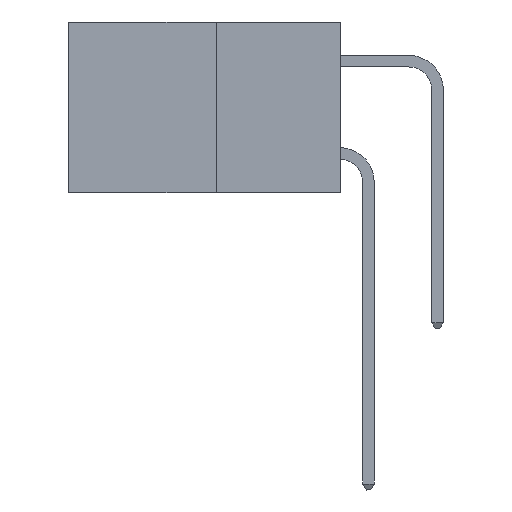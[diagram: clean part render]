
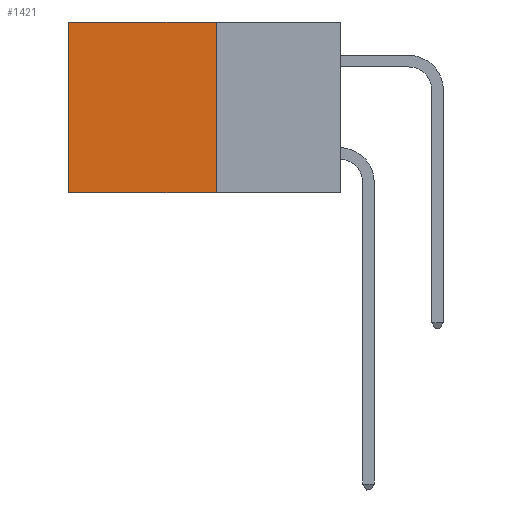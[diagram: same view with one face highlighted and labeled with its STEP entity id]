
A CAD part, left-side view. The second image highlights one B-rep face of the part: STEP entity #1421.
In plain terms, the highlighted planar face has unit normal (-1, 0, 0).
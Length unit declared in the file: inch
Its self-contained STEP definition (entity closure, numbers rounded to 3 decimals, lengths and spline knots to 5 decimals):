
#154 = DIRECTION ( 'NONE',  ( 0., 0., -1. ) ) ;
#242 = ORIENTED_EDGE ( 'NONE', *, *, #6217, .T. ) ;
#708 = FACE_OUTER_BOUND ( 'NONE', #22611, .T. ) ;
#1421 = ADVANCED_FACE ( 'NONE', ( #708 ), #15567, .F. ) ;
#2960 = CARTESIAN_POINT ( 'NONE',  ( 0.277, 0.27, 0. ) ) ;
#3631 = LINE ( 'NONE', #2960, #13345 ) ;
#5455 = ORIENTED_EDGE ( 'NONE', *, *, #10503, .T. ) ;
#5619 = CARTESIAN_POINT ( 'NONE',  ( 0.277, 0.59, -0.37 ) ) ;
#6217 = EDGE_CURVE ( 'NONE', #20292, #15551, #18264, .T. ) ;
#8264 = EDGE_CURVE ( 'NONE', #15631, #15551, #11752, .T. ) ;
#8763 = VECTOR ( 'NONE', #12217, 39.37008 ) ;
#9467 = DIRECTION ( 'NONE',  ( 0., 1., 0. ) ) ;
#10188 = CARTESIAN_POINT ( 'NONE',  ( 0.277, 0.59, 0. ) ) ;
#10309 = CARTESIAN_POINT ( 'NONE',  ( 0.277, 0.59, -0.37 ) ) ;
#10390 = CARTESIAN_POINT ( 'NONE',  ( 0.277, 0.27, -0.37 ) ) ;
#10503 = EDGE_CURVE ( 'NONE', #15727, #20292, #3631, .T. ) ;
#11217 = CARTESIAN_POINT ( 'NONE',  ( 0.277, 0.27, -0.37 ) ) ;
#11752 = LINE ( 'NONE', #11217, #20916 ) ;
#11766 = CARTESIAN_POINT ( 'NONE',  ( 0.277, 0.27, -0.37 ) ) ;
#12217 = DIRECTION ( 'NONE',  ( 0., 0., -1. ) ) ;
#13345 = VECTOR ( 'NONE', #21208, 39.37008 ) ;
#13395 = VECTOR ( 'NONE', #154, 39.37008 ) ;
#15551 = VERTEX_POINT ( 'NONE', #10309 ) ;
#15567 = PLANE ( 'NONE',  #21886 ) ;
#15631 = VERTEX_POINT ( 'NONE', #17955 ) ;
#15727 = VERTEX_POINT ( 'NONE', #21906 ) ;
#17955 = CARTESIAN_POINT ( 'NONE',  ( 0.277, 0.27, -0.37 ) ) ;
#18264 = LINE ( 'NONE', #5619, #13395 ) ;
#18292 = ORIENTED_EDGE ( 'NONE', *, *, #8264, .F. ) ;
#19075 = EDGE_CURVE ( 'NONE', #15727, #15631, #23383, .T. ) ;
#20292 = VERTEX_POINT ( 'NONE', #10188 ) ;
#20298 = ORIENTED_EDGE ( 'NONE', *, *, #19075, .F. ) ;
#20916 = VECTOR ( 'NONE', #9467, 39.37008 ) ;
#21208 = DIRECTION ( 'NONE',  ( 0., 1., 0. ) ) ;
#21281 = DIRECTION ( 'NONE',  ( 0., 0., -1. ) ) ;
#21886 = AXIS2_PLACEMENT_3D ( 'NONE', #11766, #23444, #21281 ) ;
#21906 = CARTESIAN_POINT ( 'NONE',  ( 0.277, 0.27, 0. ) ) ;
#22611 = EDGE_LOOP ( 'NONE', ( #242, #18292, #20298, #5455 ) ) ;
#23383 = LINE ( 'NONE', #10390, #8763 ) ;
#23444 = DIRECTION ( 'NONE',  ( 1., 0., 0. ) ) ;
